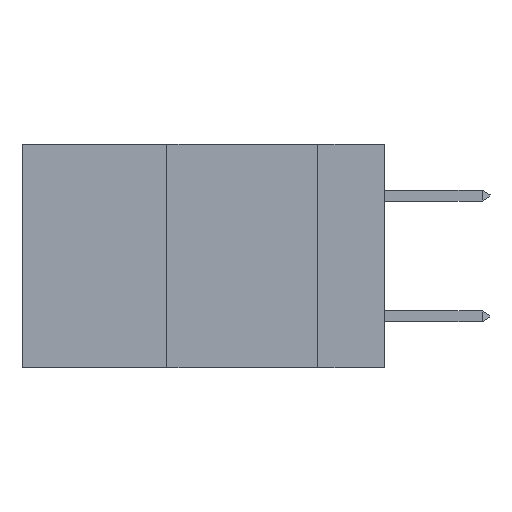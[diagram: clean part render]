
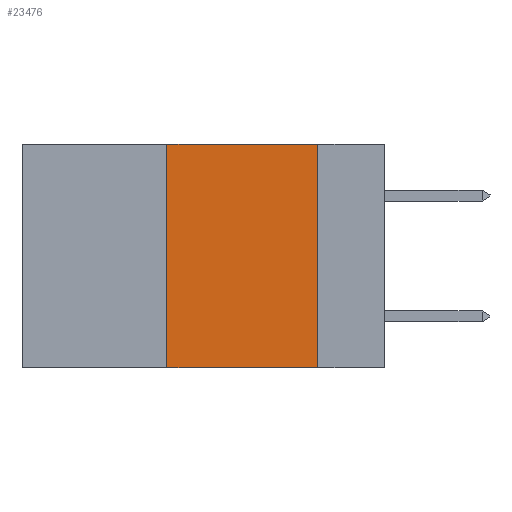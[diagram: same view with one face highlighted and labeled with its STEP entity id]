
A CAD part, left-side view. The second image highlights one B-rep face of the part: STEP entity #23476.
In plain terms, the highlighted planar face has unit normal (-1, 0, 0).
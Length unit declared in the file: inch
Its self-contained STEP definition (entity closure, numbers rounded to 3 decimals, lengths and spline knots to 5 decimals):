
#813 = VECTOR ( 'NONE', #18198, 39.37008 ) ;
#2977 = ORIENTED_EDGE ( 'NONE', *, *, #4886, .F. ) ;
#3254 = FACE_OUTER_BOUND ( 'NONE', #31959, .T. ) ;
#4886 = EDGE_CURVE ( 'NONE', #30160, #12708, #18352, .T. ) ;
#5422 = DIRECTION ( 'NONE',  ( 0., -1., 0. ) ) ;
#6894 = DIRECTION ( 'NONE',  ( 0., 0., -1. ) ) ;
#8461 = AXIS2_PLACEMENT_3D ( 'NONE', #16543, #12925, #6894 ) ;
#9939 = CARTESIAN_POINT ( 'NONE',  ( 0., 0.6, -0.37 ) ) ;
#11780 = CARTESIAN_POINT ( 'NONE',  ( 0., 0.36, 0. ) ) ;
#11819 = EDGE_CURVE ( 'NONE', #22202, #27326, #39905, .T. ) ;
#12708 = VERTEX_POINT ( 'NONE', #22314 ) ;
#12925 = DIRECTION ( 'NONE',  ( 1., 0., 0. ) ) ;
#13449 = CARTESIAN_POINT ( 'NONE',  ( 0., 0.11, 0. ) ) ;
#16543 = CARTESIAN_POINT ( 'NONE',  ( 0., 0.6, 0. ) ) ;
#17311 = LINE ( 'NONE', #40491, #23310 ) ;
#18198 = DIRECTION ( 'NONE',  ( 0., 0., 1. ) ) ;
#18323 = DIRECTION ( 'NONE',  ( 0., -1., 0. ) ) ;
#18352 = LINE ( 'NONE', #11780, #813 ) ;
#21140 = ORIENTED_EDGE ( 'NONE', *, *, #37683, .T. ) ;
#21556 = ORIENTED_EDGE ( 'NONE', *, *, #22442, .F. ) ;
#22202 = VERTEX_POINT ( 'NONE', #13449 ) ;
#22314 = CARTESIAN_POINT ( 'NONE',  ( 0., 0.36, 0. ) ) ;
#22442 = EDGE_CURVE ( 'NONE', #12708, #22202, #17311, .T. ) ;
#23310 = VECTOR ( 'NONE', #5422, 39.37008 ) ;
#23476 = ADVANCED_FACE ( 'NONE', ( #3254 ), #35198, .F. ) ;
#26884 = LINE ( 'NONE', #9939, #28363 ) ;
#27326 = VERTEX_POINT ( 'NONE', #39626 ) ;
#28363 = VECTOR ( 'NONE', #18323, 39.37008 ) ;
#30157 = ORIENTED_EDGE ( 'NONE', *, *, #11819, .F. ) ;
#30160 = VERTEX_POINT ( 'NONE', #37585 ) ;
#31959 = EDGE_LOOP ( 'NONE', ( #30157, #21556, #2977, #21140 ) ) ;
#34858 = VECTOR ( 'NONE', #38191, 39.37008 ) ;
#34965 = CARTESIAN_POINT ( 'NONE',  ( 0., 0.11, 0. ) ) ;
#35198 = PLANE ( 'NONE',  #8461 ) ;
#37585 = CARTESIAN_POINT ( 'NONE',  ( 0., 0.36, -0.37 ) ) ;
#37683 = EDGE_CURVE ( 'NONE', #30160, #27326, #26884, .T. ) ;
#38191 = DIRECTION ( 'NONE',  ( 0., 0., -1. ) ) ;
#39626 = CARTESIAN_POINT ( 'NONE',  ( 0., 0.11, -0.37 ) ) ;
#39905 = LINE ( 'NONE', #34965, #34858 ) ;
#40491 = CARTESIAN_POINT ( 'NONE',  ( 0., 0.6, 0. ) ) ;
